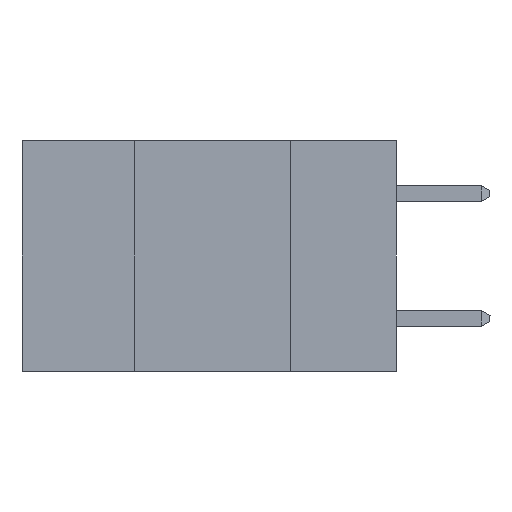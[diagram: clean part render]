
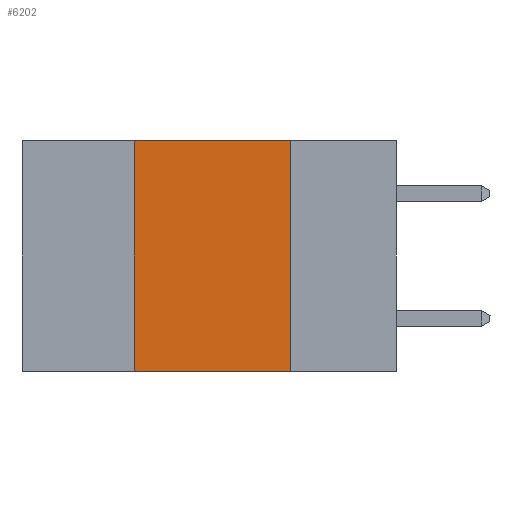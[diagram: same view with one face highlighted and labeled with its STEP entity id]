
A CAD part, left-side view. The second image highlights one B-rep face of the part: STEP entity #6202.
In plain terms, the highlighted planar face has unit normal (-1, 0, 0).
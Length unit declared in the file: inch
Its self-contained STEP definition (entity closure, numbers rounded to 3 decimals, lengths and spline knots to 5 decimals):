
#144 = CARTESIAN_POINT ( 'NONE',  ( 0., 0.42, 0. ) ) ;
#318 = VECTOR ( 'NONE', #7119, 39.37008 ) ;
#1446 = VECTOR ( 'NONE', #2159, 39.37008 ) ;
#2012 = DIRECTION ( 'NONE',  ( 0., 0., 1. ) ) ;
#2040 = FACE_OUTER_BOUND ( 'NONE', #13176, .T. ) ;
#2064 = CARTESIAN_POINT ( 'NONE',  ( 0., 0.42, -0.37 ) ) ;
#2088 = ORIENTED_EDGE ( 'NONE', *, *, #4799, .F. ) ;
#2159 = DIRECTION ( 'NONE',  ( 0., -1., 0. ) ) ;
#2173 = VECTOR ( 'NONE', #2012, 39.37008 ) ;
#2303 = CARTESIAN_POINT ( 'NONE',  ( 0., 0.6, 0. ) ) ;
#2463 = VERTEX_POINT ( 'NONE', #13974 ) ;
#3142 = CARTESIAN_POINT ( 'NONE',  ( 0., 0.42, -0.37 ) ) ;
#3714 = AXIS2_PLACEMENT_3D ( 'NONE', #11834, #11820, #11817 ) ;
#4554 = CARTESIAN_POINT ( 'NONE',  ( 0., 0.17, 0. ) ) ;
#4799 = EDGE_CURVE ( 'NONE', #7428, #2463, #12029, .T. ) ;
#5259 = LINE ( 'NONE', #2064, #2173 ) ;
#6086 = LINE ( 'NONE', #7459, #318 ) ;
#6202 = ADVANCED_FACE ( 'NONE', ( #2040 ), #11915, .F. ) ;
#7119 = DIRECTION ( 'NONE',  ( 0., -1., 0. ) ) ;
#7428 = VERTEX_POINT ( 'NONE', #4554 ) ;
#7459 = CARTESIAN_POINT ( 'NONE',  ( 0., 0.6, -0.37 ) ) ;
#7804 = EDGE_CURVE ( 'NONE', #12569, #14340, #5259, .T. ) ;
#8135 = ORIENTED_EDGE ( 'NONE', *, *, #9262, .F. ) ;
#8502 = LINE ( 'NONE', #2303, #1446 ) ;
#9154 = VECTOR ( 'NONE', #10106, 39.37008 ) ;
#9262 = EDGE_CURVE ( 'NONE', #14340, #7428, #8502, .T. ) ;
#10106 = DIRECTION ( 'NONE',  ( 0., 0., -1. ) ) ;
#11004 = CARTESIAN_POINT ( 'NONE',  ( 0., 0.17, -0.37 ) ) ;
#11817 = DIRECTION ( 'NONE',  ( 0., 0., -1. ) ) ;
#11820 = DIRECTION ( 'NONE',  ( 1., 0., 0. ) ) ;
#11834 = CARTESIAN_POINT ( 'NONE',  ( 0., 0.6, 0. ) ) ;
#11915 = PLANE ( 'NONE',  #3714 ) ;
#12029 = LINE ( 'NONE', #11004, #9154 ) ;
#12389 = ORIENTED_EDGE ( 'NONE', *, *, #13552, .T. ) ;
#12569 = VERTEX_POINT ( 'NONE', #3142 ) ;
#13176 = EDGE_LOOP ( 'NONE', ( #2088, #8135, #14121, #12389 ) ) ;
#13552 = EDGE_CURVE ( 'NONE', #12569, #2463, #6086, .T. ) ;
#13974 = CARTESIAN_POINT ( 'NONE',  ( 0., 0.17, -0.37 ) ) ;
#14121 = ORIENTED_EDGE ( 'NONE', *, *, #7804, .F. ) ;
#14340 = VERTEX_POINT ( 'NONE', #144 ) ;
